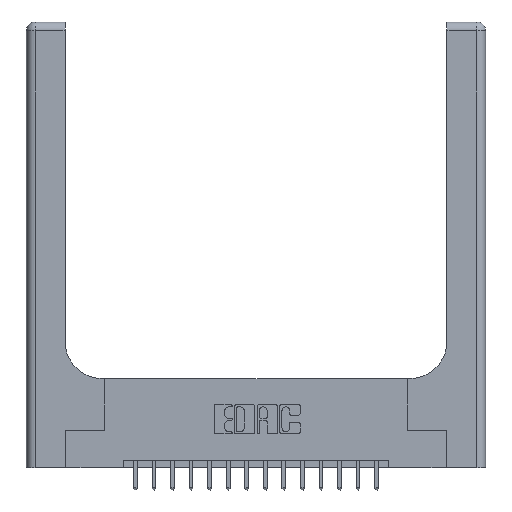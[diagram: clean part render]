
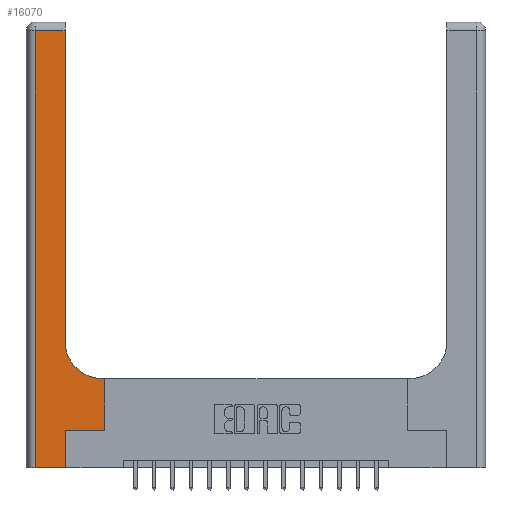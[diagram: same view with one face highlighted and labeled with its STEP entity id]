
A CAD part, top view. The second image highlights one B-rep face of the part: STEP entity #16070.
In plain terms, the highlighted planar face has unit normal (0, 0, 1).
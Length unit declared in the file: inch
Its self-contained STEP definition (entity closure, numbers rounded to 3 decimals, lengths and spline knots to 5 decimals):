
#138 = ORIENTED_EDGE ( 'NONE', *, *, #12701, .T. ) ;
#447 = LINE ( 'NONE', #9074, #9437 ) ;
#644 = DIRECTION ( 'NONE',  ( -1., 0., 0. ) ) ;
#1042 = DIRECTION ( 'NONE',  ( -1., 0., 0. ) ) ;
#1915 = VERTEX_POINT ( 'NONE', #12450 ) ;
#2015 = DIRECTION ( 'NONE',  ( 1., 0., 0. ) ) ;
#2070 = DIRECTION ( 'NONE',  ( 0., 1., 0. ) ) ;
#2126 = VECTOR ( 'NONE', #9511, 39.37008 ) ;
#2275 = LINE ( 'NONE', #17746, #2126 ) ;
#2432 = EDGE_CURVE ( 'NONE', #11570, #13031, #10353, .T. ) ;
#2556 = ORIENTED_EDGE ( 'NONE', *, *, #11525, .T. ) ;
#2816 = CARTESIAN_POINT ( 'NONE',  ( 0.51, 0.85, 0.37 ) ) ;
#3254 = VERTEX_POINT ( 'NONE', #15065 ) ;
#3493 = CIRCLE ( 'NONE', #6197, 0.25 ) ;
#4061 = VERTEX_POINT ( 'NONE', #17459 ) ;
#4432 = DIRECTION ( 'NONE',  ( 0., 0., -1. ) ) ;
#4980 = EDGE_CURVE ( 'NONE', #16920, #18098, #2275, .T. ) ;
#5365 = LINE ( 'NONE', #13892, #15302 ) ;
#5444 = EDGE_LOOP ( 'NONE', ( #9681, #7579, #9393, #16493, #138, #2556, #13115, #14872, #8993 ) ) ;
#5660 = CARTESIAN_POINT ( 'NONE',  ( 0.265, 0., 0.37 ) ) ;
#5790 = EDGE_CURVE ( 'NONE', #4061, #11570, #16863, .T. ) ;
#6051 = CARTESIAN_POINT ( 'NONE',  ( 0.26, 0.6, 0.37 ) ) ;
#6093 = PLANE ( 'NONE',  #13372 ) ;
#6197 = AXIS2_PLACEMENT_3D ( 'NONE', #2816, #4432, #16980 ) ;
#6209 = VECTOR ( 'NONE', #2070, 39.37008 ) ;
#6273 = DIRECTION ( 'NONE',  ( 0., 0., -1. ) ) ;
#6534 = DIRECTION ( 'NONE',  ( 0., 1., 0. ) ) ;
#6870 = LINE ( 'NONE', #16439, #12143 ) ;
#6909 = LINE ( 'NONE', #11208, #13336 ) ;
#6988 = EDGE_CURVE ( 'NONE', #3254, #16920, #5365, .T. ) ;
#7579 = ORIENTED_EDGE ( 'NONE', *, *, #6988, .T. ) ;
#8587 = DIRECTION ( 'NONE',  ( -1., 0., 0. ) ) ;
#8993 = ORIENTED_EDGE ( 'NONE', *, *, #11720, .T. ) ;
#9074 = CARTESIAN_POINT ( 'NONE',  ( 0., 0., 0.37 ) ) ;
#9310 = DIRECTION ( 'NONE',  ( 1., 0., 0. ) ) ;
#9391 = EDGE_CURVE ( 'NONE', #18098, #12916, #447, .T. ) ;
#9393 = ORIENTED_EDGE ( 'NONE', *, *, #4980, .T. ) ;
#9437 = VECTOR ( 'NONE', #2015, 39.37008 ) ;
#9498 = EDGE_CURVE ( 'NONE', #15911, #3254, #6909, .T. ) ;
#9511 = DIRECTION ( 'NONE',  ( 0., -1., 0. ) ) ;
#9596 = CARTESIAN_POINT ( 'NONE',  ( 0.528, 0.6, 0.37 ) ) ;
#9681 = ORIENTED_EDGE ( 'NONE', *, *, #9498, .T. ) ;
#9958 = CARTESIAN_POINT ( 'NONE',  ( 0.26, 0.85, 0.37 ) ) ;
#9969 = CARTESIAN_POINT ( 'NONE',  ( 0.51, 0.6, 0.37 ) ) ;
#10345 = CARTESIAN_POINT ( 'NONE',  ( 0.265, 0., 0.37 ) ) ;
#10353 = LINE ( 'NONE', #6051, #11483 ) ;
#11208 = CARTESIAN_POINT ( 'NONE',  ( 0.26, 3., 0.37 ) ) ;
#11483 = VECTOR ( 'NONE', #8587, 39.37008 ) ;
#11525 = EDGE_CURVE ( 'NONE', #1915, #4061, #6870, .T. ) ;
#11570 = VERTEX_POINT ( 'NONE', #9596 ) ;
#11720 = EDGE_CURVE ( 'NONE', #13031, #15911, #3493, .T. ) ;
#11885 = CARTESIAN_POINT ( 'NONE',  ( 0., 3., 0.37 ) ) ;
#11980 = FACE_OUTER_BOUND ( 'NONE', #5444, .T. ) ;
#12143 = VECTOR ( 'NONE', #9310, 39.37008 ) ;
#12450 = CARTESIAN_POINT ( 'NONE',  ( 0.265, 0.25, 0.37 ) ) ;
#12701 = EDGE_CURVE ( 'NONE', #12916, #1915, #14938, .T. ) ;
#12916 = VERTEX_POINT ( 'NONE', #5660 ) ;
#13031 = VERTEX_POINT ( 'NONE', #9969 ) ;
#13115 = ORIENTED_EDGE ( 'NONE', *, *, #5790, .T. ) ;
#13336 = VECTOR ( 'NONE', #6534, 39.37008 ) ;
#13372 = AXIS2_PLACEMENT_3D ( 'NONE', #11885, #6273, #644 ) ;
#13892 = CARTESIAN_POINT ( 'NONE',  ( 0., 2.94, 0.37 ) ) ;
#14846 = CARTESIAN_POINT ( 'NONE',  ( 0.06, 0., 0.37 ) ) ;
#14872 = ORIENTED_EDGE ( 'NONE', *, *, #2432, .T. ) ;
#14938 = LINE ( 'NONE', #10345, #6209 ) ;
#15065 = CARTESIAN_POINT ( 'NONE',  ( 0.26, 2.94, 0.37 ) ) ;
#15302 = VECTOR ( 'NONE', #1042, 39.37008 ) ;
#15541 = CARTESIAN_POINT ( 'NONE',  ( 0.06, 2.94, 0.37 ) ) ;
#15569 = VECTOR ( 'NONE', #15749, 39.37008 ) ;
#15749 = DIRECTION ( 'NONE',  ( 0., 1., 0. ) ) ;
#15911 = VERTEX_POINT ( 'NONE', #9958 ) ;
#16070 = ADVANCED_FACE ( 'NONE', ( #11980 ), #6093, .F. ) ;
#16439 = CARTESIAN_POINT ( 'NONE',  ( 0.265, 0.25, 0.37 ) ) ;
#16493 = ORIENTED_EDGE ( 'NONE', *, *, #9391, .T. ) ;
#16863 = LINE ( 'NONE', #17228, #15569 ) ;
#16920 = VERTEX_POINT ( 'NONE', #15541 ) ;
#16980 = DIRECTION ( 'NONE',  ( 1., 0., 0. ) ) ;
#17228 = CARTESIAN_POINT ( 'NONE',  ( 0.528, 0.25, 0.37 ) ) ;
#17459 = CARTESIAN_POINT ( 'NONE',  ( 0.528, 0.25, 0.37 ) ) ;
#17746 = CARTESIAN_POINT ( 'NONE',  ( 0.06, 3., 0.37 ) ) ;
#18098 = VERTEX_POINT ( 'NONE', #14846 ) ;
